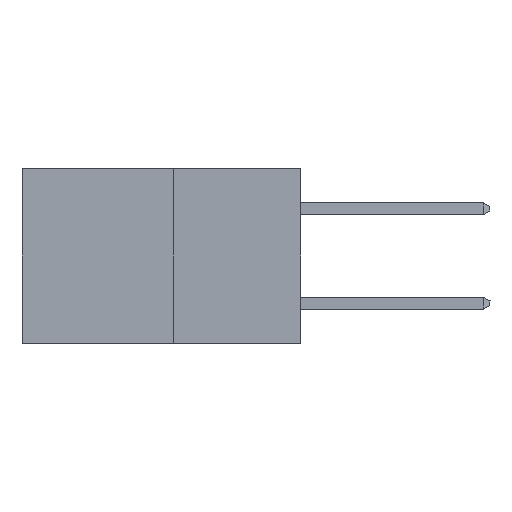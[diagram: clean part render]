
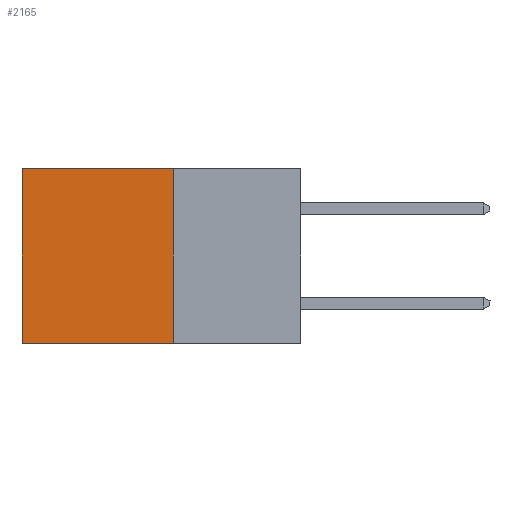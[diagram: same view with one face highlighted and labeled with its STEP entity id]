
A CAD part, left-side view. The second image highlights one B-rep face of the part: STEP entity #2165.
In plain terms, the highlighted planar face has unit normal (-1, 0, 0).
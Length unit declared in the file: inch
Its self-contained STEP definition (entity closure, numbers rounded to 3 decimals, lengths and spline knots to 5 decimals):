
#429 = VECTOR ( 'NONE', #4646, 39.37008 ) ;
#449 = DIRECTION ( 'NONE',  ( 1., 0., 0. ) ) ;
#667 = LINE ( 'NONE', #1097, #429 ) ;
#1094 = EDGE_LOOP ( 'NONE', ( #4236, #2405, #7405, #3053 ) ) ;
#1097 = CARTESIAN_POINT ( 'NONE',  ( 0.277, 0.27, -0.37 ) ) ;
#1304 = VERTEX_POINT ( 'NONE', #6937 ) ;
#1525 = DIRECTION ( 'NONE',  ( 0., 1., 0. ) ) ;
#2026 = EDGE_CURVE ( 'NONE', #8045, #4478, #4190, .T. ) ;
#2165 = ADVANCED_FACE ( 'NONE', ( #8274 ), #3620, .F. ) ;
#2178 = CARTESIAN_POINT ( 'NONE',  ( 0.277, 0.27, -0.37 ) ) ;
#2191 = VECTOR ( 'NONE', #4110, 39.37008 ) ;
#2405 = ORIENTED_EDGE ( 'NONE', *, *, #9188, .F. ) ;
#2414 = EDGE_CURVE ( 'NONE', #1304, #6468, #667, .T. ) ;
#3053 = ORIENTED_EDGE ( 'NONE', *, *, #5824, .T. ) ;
#3620 = PLANE ( 'NONE',  #4938 ) ;
#4110 = DIRECTION ( 'NONE',  ( 0., 0., -1. ) ) ;
#4134 = CARTESIAN_POINT ( 'NONE',  ( 0.277, 0.27, -0.37 ) ) ;
#4190 = LINE ( 'NONE', #5167, #2191 ) ;
#4236 = ORIENTED_EDGE ( 'NONE', *, *, #2026, .T. ) ;
#4414 = VECTOR ( 'NONE', #1525, 39.37008 ) ;
#4478 = VERTEX_POINT ( 'NONE', #5690 ) ;
#4646 = DIRECTION ( 'NONE',  ( 0., 0., -1. ) ) ;
#4766 = LINE ( 'NONE', #5266, #6453 ) ;
#4938 = AXIS2_PLACEMENT_3D ( 'NONE', #7944, #449, #5035 ) ;
#5035 = DIRECTION ( 'NONE',  ( 0., 0., -1. ) ) ;
#5167 = CARTESIAN_POINT ( 'NONE',  ( 0.277, 0.59, -0.37 ) ) ;
#5266 = CARTESIAN_POINT ( 'NONE',  ( 0.277, 0.27, 0. ) ) ;
#5690 = CARTESIAN_POINT ( 'NONE',  ( 0.277, 0.59, -0.37 ) ) ;
#5824 = EDGE_CURVE ( 'NONE', #1304, #8045, #4766, .T. ) ;
#6453 = VECTOR ( 'NONE', #7018, 39.37008 ) ;
#6468 = VERTEX_POINT ( 'NONE', #2178 ) ;
#6937 = CARTESIAN_POINT ( 'NONE',  ( 0.277, 0.27, 0. ) ) ;
#7018 = DIRECTION ( 'NONE',  ( 0., 1., 0. ) ) ;
#7405 = ORIENTED_EDGE ( 'NONE', *, *, #2414, .F. ) ;
#7944 = CARTESIAN_POINT ( 'NONE',  ( 0.277, 0.27, -0.37 ) ) ;
#8045 = VERTEX_POINT ( 'NONE', #8284 ) ;
#8186 = LINE ( 'NONE', #4134, #4414 ) ;
#8274 = FACE_OUTER_BOUND ( 'NONE', #1094, .T. ) ;
#8284 = CARTESIAN_POINT ( 'NONE',  ( 0.277, 0.59, 0. ) ) ;
#9188 = EDGE_CURVE ( 'NONE', #6468, #4478, #8186, .T. ) ;
